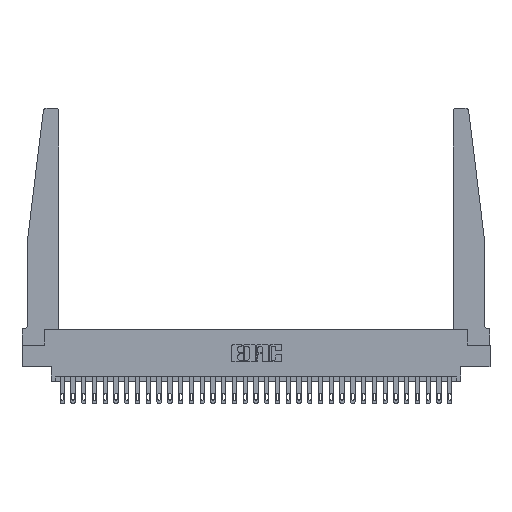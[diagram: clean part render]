
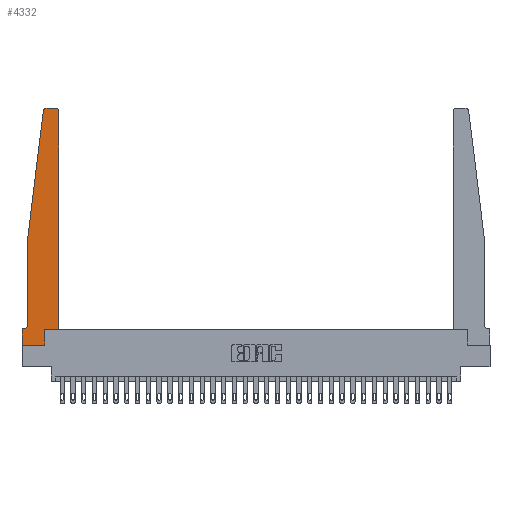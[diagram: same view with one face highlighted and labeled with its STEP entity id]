
A CAD part, top view. The second image highlights one B-rep face of the part: STEP entity #4332.
In plain terms, the highlighted planar face has unit normal (0, 0, 1).
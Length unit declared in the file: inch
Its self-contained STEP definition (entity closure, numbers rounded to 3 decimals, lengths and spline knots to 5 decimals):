
#191 = DIRECTION ( 'NONE',  ( 0., 0., 1. ) ) ;
#512 = ORIENTED_EDGE ( 'NONE', *, *, #22207, .T. ) ;
#793 = EDGE_CURVE ( 'NONE', #20830, #28272, #22577, .T. ) ;
#1869 = CARTESIAN_POINT ( 'NONE',  ( 0.27653, 2.72, 0.37 ) ) ;
#2322 = DIRECTION ( 'NONE',  ( 1., 0., 0. ) ) ;
#2328 = LINE ( 'NONE', #11599, #13562 ) ;
#2432 = VERTEX_POINT ( 'NONE', #12518 ) ;
#3437 = DIRECTION ( 'NONE',  ( 1., 0., 0. ) ) ;
#4156 = DIRECTION ( 'NONE',  ( 0., 0., -1. ) ) ;
#4332 = ADVANCED_FACE ( 'NONE', ( #12625 ), #21950, .T. ) ;
#4911 = ORIENTED_EDGE ( 'NONE', *, *, #19688, .T. ) ;
#4970 = VERTEX_POINT ( 'NONE', #14078 ) ;
#5390 = VERTEX_POINT ( 'NONE', #8429 ) ;
#5873 = EDGE_CURVE ( 'NONE', #28272, #25984, #9102, .T. ) ;
#6070 = VECTOR ( 'NONE', #13443, 39.37008 ) ;
#6101 = CARTESIAN_POINT ( 'NONE',  ( 0.065, 0.1875, 0.37 ) ) ;
#6159 = CARTESIAN_POINT ( 'NONE',  ( 0.425, 0.18, 0.37 ) ) ;
#6264 = DIRECTION ( 'NONE',  ( -1., 0., 0. ) ) ;
#7716 = VERTEX_POINT ( 'NONE', #25208 ) ;
#7819 = LINE ( 'NONE', #29027, #8425 ) ;
#8052 = DIRECTION ( 'NONE',  ( 0., 0., 1. ) ) ;
#8425 = VECTOR ( 'NONE', #17411, 39.37008 ) ;
#8429 = CARTESIAN_POINT ( 'NONE',  ( 0.065, 1.25, 0.37 ) ) ;
#8628 = ORIENTED_EDGE ( 'NONE', *, *, #12571, .T. ) ;
#9102 = LINE ( 'NONE', #18423, #27716 ) ;
#9312 = EDGE_CURVE ( 'NONE', #19942, #14032, #17369, .T. ) ;
#9479 = DIRECTION ( 'NONE',  ( 0., -1., 0. ) ) ;
#9553 = CIRCLE ( 'NONE', #29557, 0.03 ) ;
#10493 = VECTOR ( 'NONE', #15700, 39.37008 ) ;
#10660 = CARTESIAN_POINT ( 'NONE',  ( 0.015, 0.1875, 0.37 ) ) ;
#10735 = LINE ( 'NONE', #6159, #22808 ) ;
#10847 = CARTESIAN_POINT ( 'NONE',  ( 0.015, 0.2375, 0.37 ) ) ;
#10909 = CARTESIAN_POINT ( 'NONE',  ( 0., 0.1875, 0.37 ) ) ;
#11085 = DIRECTION ( 'NONE',  ( 0., 1., 0. ) ) ;
#11142 = EDGE_LOOP ( 'NONE', ( #4911, #24416, #20371, #13674, #16508, #28655, #17832, #24576, #12380, #16182, #512, #8628 ) ) ;
#11599 = CARTESIAN_POINT ( 'NONE',  ( 0.425, 0.18, 0.37 ) ) ;
#12369 = CARTESIAN_POINT ( 'NONE',  ( 0.27653, 2.75, 0.37 ) ) ;
#12380 = ORIENTED_EDGE ( 'NONE', *, *, #9312, .T. ) ;
#12518 = CARTESIAN_POINT ( 'NONE',  ( 0.065, 0.2375, 0.37 ) ) ;
#12571 = EDGE_CURVE ( 'NONE', #7716, #13323, #16698, .T. ) ;
#12625 = FACE_OUTER_BOUND ( 'NONE', #11142, .T. ) ;
#12700 = LINE ( 'NONE', #29187, #25517 ) ;
#12862 = CARTESIAN_POINT ( 'NONE',  ( 0.065, 1.25, 0.37 ) ) ;
#13092 = CARTESIAN_POINT ( 'NONE',  ( 0.25, 2.75, 0.37 ) ) ;
#13323 = VERTEX_POINT ( 'NONE', #16998 ) ;
#13427 = EDGE_CURVE ( 'NONE', #5390, #2432, #25079, .T. ) ;
#13443 = DIRECTION ( 'NONE',  ( 0., -1., 0. ) ) ;
#13562 = VECTOR ( 'NONE', #20901, 39.37008 ) ;
#13674 = ORIENTED_EDGE ( 'NONE', *, *, #13427, .T. ) ;
#13993 = CIRCLE ( 'NONE', #21338, 0.05 ) ;
#14032 = VERTEX_POINT ( 'NONE', #25341 ) ;
#14078 = CARTESIAN_POINT ( 'NONE',  ( 0.24675, 2.72367, 0.37 ) ) ;
#14335 = CARTESIAN_POINT ( 'NONE',  ( 0., 0., 0.37 ) ) ;
#14764 = EDGE_CURVE ( 'NONE', #25984, #19942, #12700, .T. ) ;
#14853 = CARTESIAN_POINT ( 'NONE',  ( 0.425, 0.18, 0.37 ) ) ;
#14890 = CARTESIAN_POINT ( 'NONE',  ( 0.2605, 0., 0.37 ) ) ;
#15700 = DIRECTION ( 'NONE',  ( -1., 0., 0. ) ) ;
#15808 = DIRECTION ( 'NONE',  ( 0., 0., 1. ) ) ;
#16182 = ORIENTED_EDGE ( 'NONE', *, *, #21731, .T. ) ;
#16508 = ORIENTED_EDGE ( 'NONE', *, *, #19307, .T. ) ;
#16546 = EDGE_CURVE ( 'NONE', #20637, #4970, #9553, .T. ) ;
#16698 = CIRCLE ( 'NONE', #20605, 0.03 ) ;
#16998 = CARTESIAN_POINT ( 'NONE',  ( 0.395, 2.75, 0.37 ) ) ;
#17369 = LINE ( 'NONE', #17667, #29433 ) ;
#17411 = DIRECTION ( 'NONE',  ( -0.122, -0.992, 0. ) ) ;
#17667 = CARTESIAN_POINT ( 'NONE',  ( 0.2605, 0.18, 0.37 ) ) ;
#17832 = ORIENTED_EDGE ( 'NONE', *, *, #5873, .T. ) ;
#18140 = LINE ( 'NONE', #13092, #29616 ) ;
#18423 = CARTESIAN_POINT ( 'NONE',  ( 0., 0., 0.37 ) ) ;
#19307 = EDGE_CURVE ( 'NONE', #2432, #20830, #13993, .T. ) ;
#19632 = CARTESIAN_POINT ( 'NONE',  ( 0., 0.1875, 0.37 ) ) ;
#19688 = EDGE_CURVE ( 'NONE', #13323, #20637, #18140, .T. ) ;
#19942 = VERTEX_POINT ( 'NONE', #14890 ) ;
#20371 = ORIENTED_EDGE ( 'NONE', *, *, #29223, .T. ) ;
#20389 = DIRECTION ( 'NONE',  ( 1., 0., 0. ) ) ;
#20431 = VERTEX_POINT ( 'NONE', #14853 ) ;
#20572 = DIRECTION ( 'NONE',  ( -1., 0., 0. ) ) ;
#20605 = AXIS2_PLACEMENT_3D ( 'NONE', #27579, #15808, #20389 ) ;
#20637 = VERTEX_POINT ( 'NONE', #12369 ) ;
#20830 = VERTEX_POINT ( 'NONE', #10660 ) ;
#20901 = DIRECTION ( 'NONE',  ( 0., 1., 0. ) ) ;
#21338 = AXIS2_PLACEMENT_3D ( 'NONE', #10847, #4156, #6264 ) ;
#21731 = EDGE_CURVE ( 'NONE', #14032, #20431, #10735, .T. ) ;
#21950 = PLANE ( 'NONE',  #28699 ) ;
#22207 = EDGE_CURVE ( 'NONE', #20431, #7716, #2328, .T. ) ;
#22577 = LINE ( 'NONE', #6101, #10493 ) ;
#22808 = VECTOR ( 'NONE', #29213, 39.37008 ) ;
#23276 = DIRECTION ( 'NONE',  ( 1., 0., 0. ) ) ;
#24416 = ORIENTED_EDGE ( 'NONE', *, *, #16546, .T. ) ;
#24576 = ORIENTED_EDGE ( 'NONE', *, *, #14764, .T. ) ;
#25079 = LINE ( 'NONE', #12862, #6070 ) ;
#25208 = CARTESIAN_POINT ( 'NONE',  ( 0.425, 2.72, 0.37 ) ) ;
#25341 = CARTESIAN_POINT ( 'NONE',  ( 0.2605, 0.18, 0.37 ) ) ;
#25517 = VECTOR ( 'NONE', #3437, 39.37008 ) ;
#25984 = VERTEX_POINT ( 'NONE', #14335 ) ;
#27579 = CARTESIAN_POINT ( 'NONE',  ( 0.395, 2.72, 0.37 ) ) ;
#27716 = VECTOR ( 'NONE', #9479, 39.37008 ) ;
#28272 = VERTEX_POINT ( 'NONE', #10909 ) ;
#28655 = ORIENTED_EDGE ( 'NONE', *, *, #793, .T. ) ;
#28699 = AXIS2_PLACEMENT_3D ( 'NONE', #19632, #8052, #23276 ) ;
#29027 = CARTESIAN_POINT ( 'NONE',  ( 0.065, 1.25, 0.37 ) ) ;
#29187 = CARTESIAN_POINT ( 'NONE',  ( 0., 0., 0.37 ) ) ;
#29213 = DIRECTION ( 'NONE',  ( 1., 0., 0. ) ) ;
#29223 = EDGE_CURVE ( 'NONE', #4970, #5390, #7819, .T. ) ;
#29433 = VECTOR ( 'NONE', #11085, 39.37008 ) ;
#29557 = AXIS2_PLACEMENT_3D ( 'NONE', #1869, #191, #2322 ) ;
#29616 = VECTOR ( 'NONE', #20572, 39.37008 ) ;
